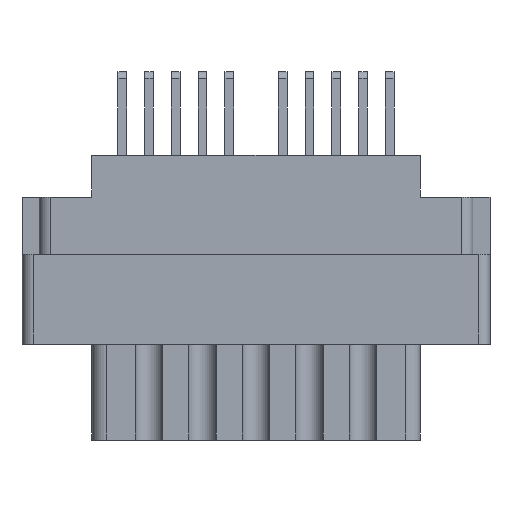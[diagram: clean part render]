
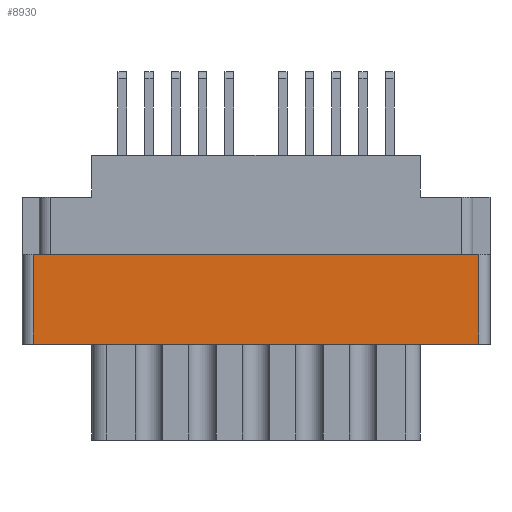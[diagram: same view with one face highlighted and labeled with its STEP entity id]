
A CAD part, front view. The second image highlights one B-rep face of the part: STEP entity #8930.
In plain terms, the highlighted planar face has unit normal (0, -1, 0).
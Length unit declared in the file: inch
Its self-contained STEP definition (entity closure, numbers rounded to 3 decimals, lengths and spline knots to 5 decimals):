
#967 = ORIENTED_EDGE ( 'NONE', *, *, #23372, .F. ) ;
#2013 = LINE ( 'NONE', #27768, #25508 ) ;
#2128 = EDGE_CURVE ( 'NONE', #19008, #11585, #4542, .T. ) ;
#4093 = ORIENTED_EDGE ( 'NONE', *, *, #24992, .T. ) ;
#4542 = LINE ( 'NONE', #13411, #23013 ) ;
#6695 = CARTESIAN_POINT ( 'NONE',  ( 0.624, -0.343, -0.798 ) ) ;
#7193 = FACE_OUTER_BOUND ( 'NONE', #28153, .T. ) ;
#7541 = CARTESIAN_POINT ( 'NONE',  ( 0.624, -0.343, -0.529 ) ) ;
#8930 = ADVANCED_FACE ( 'NONE', ( #7193 ), #20348, .T. ) ;
#9248 = EDGE_CURVE ( 'NONE', #26907, #11585, #26306, .T. ) ;
#10083 = VECTOR ( 'NONE', #11142, 39.37008 ) ;
#11142 = DIRECTION ( 'NONE',  ( 0., 0., 1. ) ) ;
#11585 = VERTEX_POINT ( 'NONE', #23078 ) ;
#11625 = CARTESIAN_POINT ( 'NONE',  ( -0.656, -0.343, -0.798 ) ) ;
#11629 = CARTESIAN_POINT ( 'NONE',  ( -0.624, -0.343, -0.277 ) ) ;
#13411 = CARTESIAN_POINT ( 'NONE',  ( 0., -0.343, -0.277 ) ) ;
#15208 = ORIENTED_EDGE ( 'NONE', *, *, #9248, .T. ) ;
#15229 = LINE ( 'NONE', #25664, #26364 ) ;
#15794 = DIRECTION ( 'NONE',  ( 0., 0., -1. ) ) ;
#18881 = ORIENTED_EDGE ( 'NONE', *, *, #2128, .F. ) ;
#19008 = VERTEX_POINT ( 'NONE', #11629 ) ;
#20348 = PLANE ( 'NONE',  #21486 ) ;
#21219 = DIRECTION ( 'NONE',  ( -1., 0., 0. ) ) ;
#21486 = AXIS2_PLACEMENT_3D ( 'NONE', #11625, #24790, #15794 ) ;
#23013 = VECTOR ( 'NONE', #28136, 39.37008 ) ;
#23078 = CARTESIAN_POINT ( 'NONE',  ( 0.624, -0.343, -0.277 ) ) ;
#23372 = EDGE_CURVE ( 'NONE', #26907, #26076, #15229, .T. ) ;
#23773 = CARTESIAN_POINT ( 'NONE',  ( -0.624, -0.343, -0.529 ) ) ;
#24790 = DIRECTION ( 'NONE',  ( 0., -1., 0. ) ) ;
#24992 = EDGE_CURVE ( 'NONE', #19008, #26076, #2013, .T. ) ;
#25508 = VECTOR ( 'NONE', #28054, 39.37008 ) ;
#25664 = CARTESIAN_POINT ( 'NONE',  ( 0., -0.343, -0.529 ) ) ;
#26076 = VERTEX_POINT ( 'NONE', #23773 ) ;
#26306 = LINE ( 'NONE', #6695, #10083 ) ;
#26364 = VECTOR ( 'NONE', #21219, 39.37008 ) ;
#26907 = VERTEX_POINT ( 'NONE', #7541 ) ;
#27768 = CARTESIAN_POINT ( 'NONE',  ( -0.624, -0.343, -0.798 ) ) ;
#28054 = DIRECTION ( 'NONE',  ( 0., 0., -1. ) ) ;
#28136 = DIRECTION ( 'NONE',  ( 1., 0., 0. ) ) ;
#28153 = EDGE_LOOP ( 'NONE', ( #18881, #4093, #967, #15208 ) ) ;
